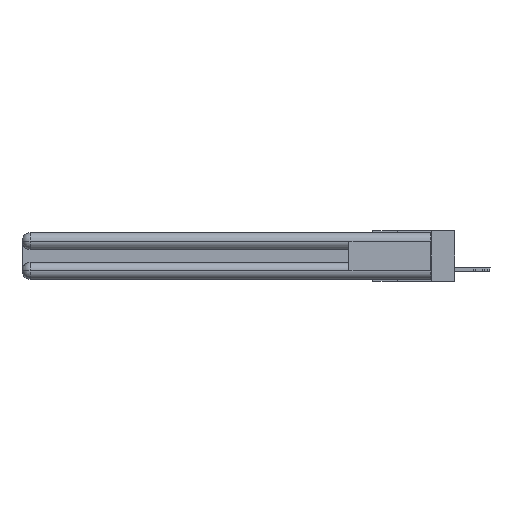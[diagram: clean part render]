
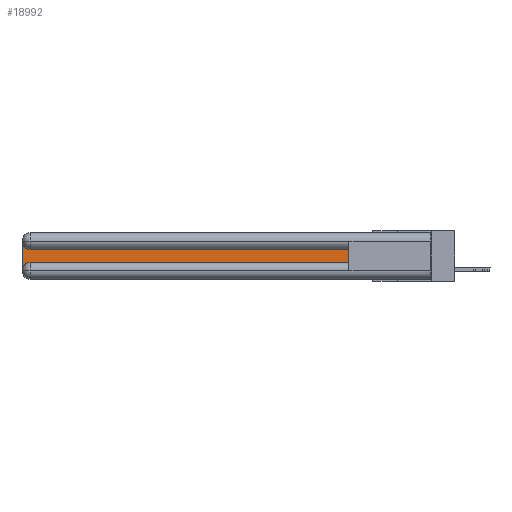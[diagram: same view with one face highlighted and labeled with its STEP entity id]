
A CAD part, left-side view. The second image highlights one B-rep face of the part: STEP entity #18992.
In plain terms, the highlighted planar face has unit normal (-1, 0, 0).
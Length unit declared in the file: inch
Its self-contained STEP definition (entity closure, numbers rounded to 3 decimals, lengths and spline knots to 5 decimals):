
#36 = VERTEX_POINT ( 'NONE', #22191 ) ;
#328 = LINE ( 'NONE', #8072, #17718 ) ;
#861 = DIRECTION ( 'NONE',  ( 0., 0., -1. ) ) ;
#2645 = DIRECTION ( 'NONE',  ( 1., 0., 0. ) ) ;
#2735 = ORIENTED_EDGE ( 'NONE', *, *, #14082, .T. ) ;
#3111 = LINE ( 'NONE', #13261, #11794 ) ;
#3604 = VECTOR ( 'NONE', #21586, 39.37008 ) ;
#4783 = CARTESIAN_POINT ( 'NONE',  ( 0.075, 0.6, -0.1225 ) ) ;
#4835 = DIRECTION ( 'NONE',  ( 1., 0., 0. ) ) ;
#5074 = VECTOR ( 'NONE', #27012, 39.37008 ) ;
#6421 = EDGE_LOOP ( 'NONE', ( #2735, #24942, #17265, #11191, #24098, #27425 ) ) ;
#7211 = CARTESIAN_POINT ( 'NONE',  ( 0.075, 2.94, -0.2775 ) ) ;
#7795 = EDGE_CURVE ( 'NONE', #8795, #19042, #328, .T. ) ;
#8072 = CARTESIAN_POINT ( 'NONE',  ( 0.075, 0.6, -0.2175 ) ) ;
#8447 = LINE ( 'NONE', #26344, #5074 ) ;
#8795 = VERTEX_POINT ( 'NONE', #24555 ) ;
#10063 = AXIS2_PLACEMENT_3D ( 'NONE', #17857, #4835, #26520 ) ;
#10171 = EDGE_CURVE ( 'NONE', #24012, #10639, #20272, .T. ) ;
#10262 = CIRCLE ( 'NONE', #10063, 0.06 ) ;
#10393 = DIRECTION ( 'NONE',  ( 0., 0., 1. ) ) ;
#10639 = VERTEX_POINT ( 'NONE', #11873 ) ;
#11143 = DIRECTION ( 'NONE',  ( 1., 0., 0. ) ) ;
#11162 = CARTESIAN_POINT ( 'NONE',  ( 0.075, 0.6, -0.2175 ) ) ;
#11191 = ORIENTED_EDGE ( 'NONE', *, *, #10171, .T. ) ;
#11246 = PLANE ( 'NONE',  #26444 ) ;
#11794 = VECTOR ( 'NONE', #17735, 39.37008 ) ;
#11873 = CARTESIAN_POINT ( 'NONE',  ( 0.075, 2.94, -0.2175 ) ) ;
#13116 = CARTESIAN_POINT ( 'NONE',  ( 0.075, 3., -0.0625 ) ) ;
#13261 = CARTESIAN_POINT ( 'NONE',  ( 0.075, 0.6, -0.1225 ) ) ;
#14082 = EDGE_CURVE ( 'NONE', #19042, #36, #3111, .T. ) ;
#16028 = VERTEX_POINT ( 'NONE', #13116 ) ;
#16226 = FACE_OUTER_BOUND ( 'NONE', #6421, .T. ) ;
#17265 = ORIENTED_EDGE ( 'NONE', *, *, #20108, .T. ) ;
#17674 = EDGE_CURVE ( 'NONE', #10639, #8795, #26731, .T. ) ;
#17718 = VECTOR ( 'NONE', #10393, 39.37008 ) ;
#17735 = DIRECTION ( 'NONE',  ( 0., 1., 0. ) ) ;
#17857 = CARTESIAN_POINT ( 'NONE',  ( 0.075, 2.94, -0.0625 ) ) ;
#18992 = ADVANCED_FACE ( 'NONE', ( #16226 ), #11246, .F. ) ;
#19042 = VERTEX_POINT ( 'NONE', #4783 ) ;
#20108 = EDGE_CURVE ( 'NONE', #16028, #24012, #8447, .T. ) ;
#20272 = CIRCLE ( 'NONE', #26494, 0.06 ) ;
#20363 = CARTESIAN_POINT ( 'NONE',  ( 0.075, 3., -0.2775 ) ) ;
#21586 = DIRECTION ( 'NONE',  ( 0., -1., 0. ) ) ;
#21870 = CARTESIAN_POINT ( 'NONE',  ( 0.075, 3., -0.1225 ) ) ;
#21951 = DIRECTION ( 'NONE',  ( 0., 0., -1. ) ) ;
#22191 = CARTESIAN_POINT ( 'NONE',  ( 0.075, 2.94, -0.1225 ) ) ;
#24012 = VERTEX_POINT ( 'NONE', #20363 ) ;
#24098 = ORIENTED_EDGE ( 'NONE', *, *, #17674, .T. ) ;
#24555 = CARTESIAN_POINT ( 'NONE',  ( 0.075, 0.6, -0.2175 ) ) ;
#24942 = ORIENTED_EDGE ( 'NONE', *, *, #26045, .T. ) ;
#26045 = EDGE_CURVE ( 'NONE', #36, #16028, #10262, .T. ) ;
#26344 = CARTESIAN_POINT ( 'NONE',  ( 0.075, 3., -0.2175 ) ) ;
#26444 = AXIS2_PLACEMENT_3D ( 'NONE', #21870, #2645, #21951 ) ;
#26494 = AXIS2_PLACEMENT_3D ( 'NONE', #7211, #11143, #861 ) ;
#26520 = DIRECTION ( 'NONE',  ( 0., 0., -1. ) ) ;
#26731 = LINE ( 'NONE', #11162, #3604 ) ;
#27012 = DIRECTION ( 'NONE',  ( 0., 0., -1. ) ) ;
#27425 = ORIENTED_EDGE ( 'NONE', *, *, #7795, .T. ) ;
